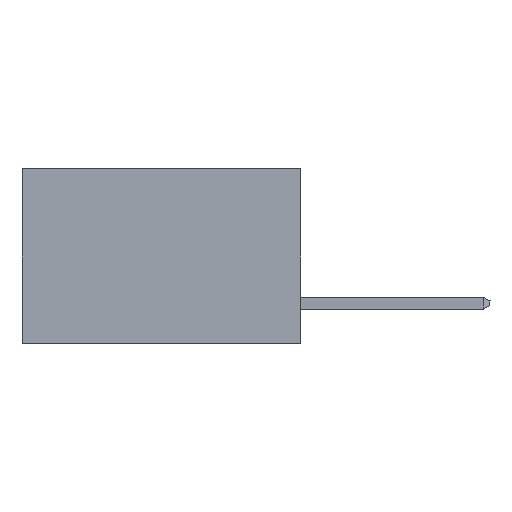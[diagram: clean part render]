
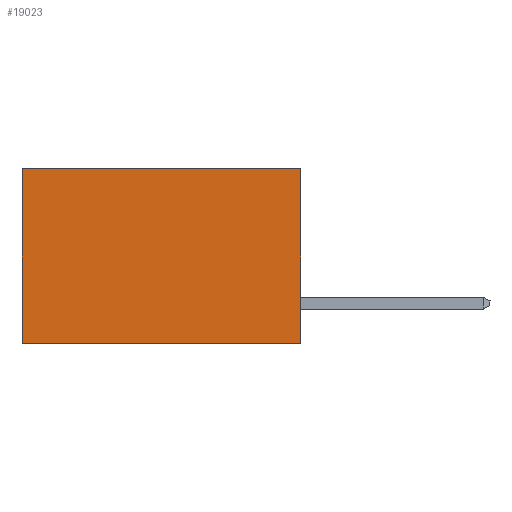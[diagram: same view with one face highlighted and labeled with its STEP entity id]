
A CAD part, left-side view. The second image highlights one B-rep face of the part: STEP entity #19023.
In plain terms, the highlighted planar face has unit normal (-1, 0, 0).
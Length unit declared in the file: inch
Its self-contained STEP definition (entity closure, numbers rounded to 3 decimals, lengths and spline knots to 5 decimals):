
#135 = LINE ( 'NONE', #20201, #6076 ) ;
#4588 = ORIENTED_EDGE ( 'NONE', *, *, #9892, .T. ) ;
#4620 = DIRECTION ( 'NONE',  ( 0., 0., -1. ) ) ;
#5087 = EDGE_CURVE ( 'NONE', #17977, #22314, #14644, .T. ) ;
#6076 = VECTOR ( 'NONE', #13887, 39.37008 ) ;
#6315 = CARTESIAN_POINT ( 'NONE',  ( 0.277, 0.59, -0.37 ) ) ;
#6619 = CARTESIAN_POINT ( 'NONE',  ( 0.277, 0.59, -0.37 ) ) ;
#7737 = CARTESIAN_POINT ( 'NONE',  ( 0.277, 0.59, 0. ) ) ;
#8070 = VECTOR ( 'NONE', #4620, 39.37008 ) ;
#8525 = AXIS2_PLACEMENT_3D ( 'NONE', #11643, #27086, #13875 ) ;
#8811 = LINE ( 'NONE', #9116, #19144 ) ;
#9113 = ORIENTED_EDGE ( 'NONE', *, *, #13844, .F. ) ;
#9116 = CARTESIAN_POINT ( 'NONE',  ( 0.277, 0., -0.37 ) ) ;
#9892 = EDGE_CURVE ( 'NONE', #24195, #17977, #135, .T. ) ;
#10240 = VERTEX_POINT ( 'NONE', #11262 ) ;
#11262 = CARTESIAN_POINT ( 'NONE',  ( 0.277, 0., -0.37 ) ) ;
#11448 = VECTOR ( 'NONE', #21450, 39.37008 ) ;
#11643 = CARTESIAN_POINT ( 'NONE',  ( 0.277, 0., -0.37 ) ) ;
#12145 = LINE ( 'NONE', #23677, #11448 ) ;
#13844 = EDGE_CURVE ( 'NONE', #24195, #10240, #8811, .T. ) ;
#13875 = DIRECTION ( 'NONE',  ( 0., 0., -1. ) ) ;
#13887 = DIRECTION ( 'NONE',  ( 0., 1., 0. ) ) ;
#14644 = LINE ( 'NONE', #6315, #8070 ) ;
#17977 = VERTEX_POINT ( 'NONE', #7737 ) ;
#19023 = ADVANCED_FACE ( 'NONE', ( #21856 ), #24871, .F. ) ;
#19144 = VECTOR ( 'NONE', #22308, 39.37008 ) ;
#20201 = CARTESIAN_POINT ( 'NONE',  ( 0.277, 0., 0. ) ) ;
#20887 = EDGE_CURVE ( 'NONE', #10240, #22314, #12145, .T. ) ;
#21450 = DIRECTION ( 'NONE',  ( 0., 1., 0. ) ) ;
#21856 = FACE_OUTER_BOUND ( 'NONE', #24838, .T. ) ;
#22253 = CARTESIAN_POINT ( 'NONE',  ( 0.277, 0., 0. ) ) ;
#22308 = DIRECTION ( 'NONE',  ( 0., 0., -1. ) ) ;
#22314 = VERTEX_POINT ( 'NONE', #6619 ) ;
#23677 = CARTESIAN_POINT ( 'NONE',  ( 0.277, 0., -0.37 ) ) ;
#24195 = VERTEX_POINT ( 'NONE', #22253 ) ;
#24838 = EDGE_LOOP ( 'NONE', ( #26856, #27246, #9113, #4588 ) ) ;
#24871 = PLANE ( 'NONE',  #8525 ) ;
#26856 = ORIENTED_EDGE ( 'NONE', *, *, #5087, .T. ) ;
#27086 = DIRECTION ( 'NONE',  ( 1., 0., 0. ) ) ;
#27246 = ORIENTED_EDGE ( 'NONE', *, *, #20887, .F. ) ;
